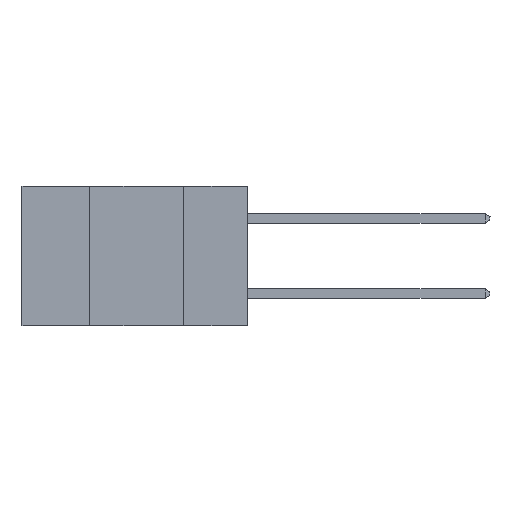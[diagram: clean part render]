
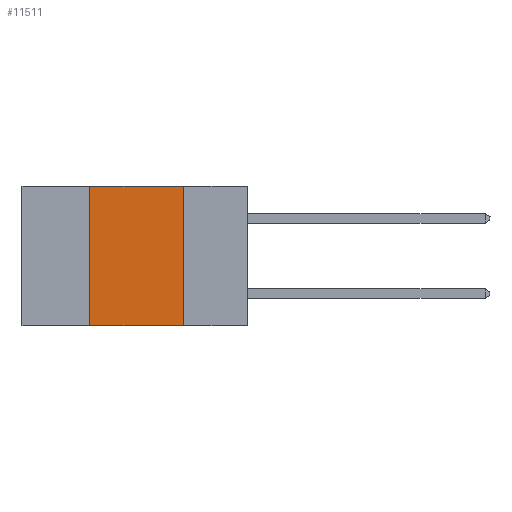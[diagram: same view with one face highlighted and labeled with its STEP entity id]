
A CAD part, left-side view. The second image highlights one B-rep face of the part: STEP entity #11511.
In plain terms, the highlighted planar face has unit normal (-1, 0, 0).
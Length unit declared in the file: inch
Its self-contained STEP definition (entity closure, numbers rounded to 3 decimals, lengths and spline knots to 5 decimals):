
#578 = CARTESIAN_POINT ( 'NONE',  ( 0., 0.6, 0. ) ) ;
#829 = CARTESIAN_POINT ( 'NONE',  ( 0., 0.6, 0. ) ) ;
#2346 = VERTEX_POINT ( 'NONE', #16472 ) ;
#3014 = ORIENTED_EDGE ( 'NONE', *, *, #4121, .F. ) ;
#4121 = EDGE_CURVE ( 'NONE', #14736, #10609, #4278, .T. ) ;
#4278 = LINE ( 'NONE', #20239, #18822 ) ;
#5006 = DIRECTION ( 'NONE',  ( 0., -1., 0. ) ) ;
#5372 = ORIENTED_EDGE ( 'NONE', *, *, #14191, .F. ) ;
#5428 = LINE ( 'NONE', #13425, #19853 ) ;
#6520 = CARTESIAN_POINT ( 'NONE',  ( 0., 0.17, -0.37 ) ) ;
#6846 = DIRECTION ( 'NONE',  ( 1., 0., 0. ) ) ;
#9617 = DIRECTION ( 'NONE',  ( 0., -1., 0. ) ) ;
#10038 = DIRECTION ( 'NONE',  ( 0., 0., -1. ) ) ;
#10609 = VERTEX_POINT ( 'NONE', #6520 ) ;
#11307 = EDGE_LOOP ( 'NONE', ( #3014, #5372, #16013, #25732 ) ) ;
#11511 = ADVANCED_FACE ( 'NONE', ( #20705 ), #18753, .F. ) ;
#11918 = CARTESIAN_POINT ( 'NONE',  ( 0., 0.17, 0. ) ) ;
#11980 = VECTOR ( 'NONE', #5006, 39.37008 ) ;
#12109 = CARTESIAN_POINT ( 'NONE',  ( 0., 0.42, -0.37 ) ) ;
#12504 = EDGE_CURVE ( 'NONE', #18557, #10609, #5428, .T. ) ;
#12586 = EDGE_CURVE ( 'NONE', #18557, #2346, #13955, .T. ) ;
#13141 = AXIS2_PLACEMENT_3D ( 'NONE', #829, #6846, #14844 ) ;
#13425 = CARTESIAN_POINT ( 'NONE',  ( 0., 0.6, -0.37 ) ) ;
#13955 = LINE ( 'NONE', #12109, #25699 ) ;
#14080 = DIRECTION ( 'NONE',  ( 0., 0., 1. ) ) ;
#14191 = EDGE_CURVE ( 'NONE', #2346, #14736, #22919, .T. ) ;
#14736 = VERTEX_POINT ( 'NONE', #11918 ) ;
#14844 = DIRECTION ( 'NONE',  ( 0., 0., -1. ) ) ;
#16013 = ORIENTED_EDGE ( 'NONE', *, *, #12586, .F. ) ;
#16472 = CARTESIAN_POINT ( 'NONE',  ( 0., 0.42, 0. ) ) ;
#18557 = VERTEX_POINT ( 'NONE', #21643 ) ;
#18753 = PLANE ( 'NONE',  #13141 ) ;
#18822 = VECTOR ( 'NONE', #10038, 39.37008 ) ;
#19853 = VECTOR ( 'NONE', #9617, 39.37008 ) ;
#20239 = CARTESIAN_POINT ( 'NONE',  ( 0., 0.17, -0.37 ) ) ;
#20705 = FACE_OUTER_BOUND ( 'NONE', #11307, .T. ) ;
#21643 = CARTESIAN_POINT ( 'NONE',  ( 0., 0.42, -0.37 ) ) ;
#22919 = LINE ( 'NONE', #578, #11980 ) ;
#25699 = VECTOR ( 'NONE', #14080, 39.37008 ) ;
#25732 = ORIENTED_EDGE ( 'NONE', *, *, #12504, .T. ) ;
